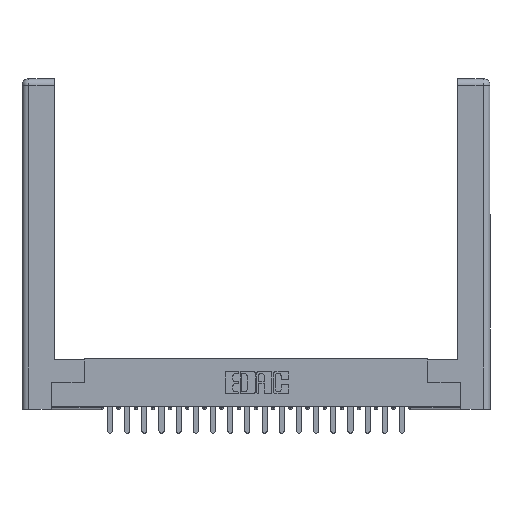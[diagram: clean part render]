
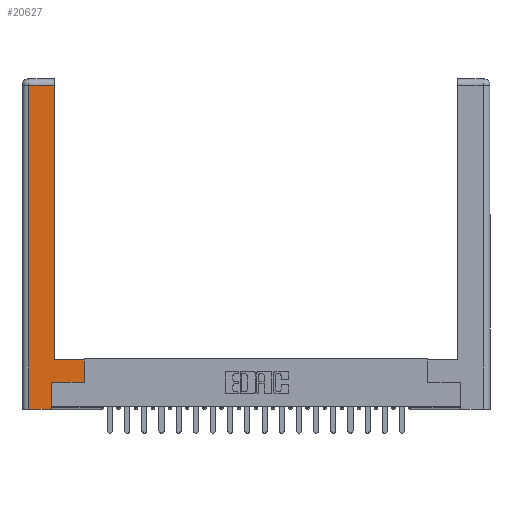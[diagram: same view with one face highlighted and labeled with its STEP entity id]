
A CAD part, top view. The second image highlights one B-rep face of the part: STEP entity #20627.
In plain terms, the highlighted planar face has unit normal (0, 0, 1).
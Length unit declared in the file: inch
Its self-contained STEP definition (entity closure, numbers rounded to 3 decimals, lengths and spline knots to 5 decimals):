
#441 = EDGE_CURVE ( 'NONE', #831, #10784, #10107, .T. ) ;
#831 = VERTEX_POINT ( 'NONE', #1088 ) ;
#875 = VERTEX_POINT ( 'NONE', #9645 ) ;
#1088 = CARTESIAN_POINT ( 'NONE',  ( 0.265, 0., 0. ) ) ;
#1110 = DIRECTION ( 'NONE',  ( 0., 1., 0. ) ) ;
#1172 = CARTESIAN_POINT ( 'NONE',  ( 0.295, 2.94, 0. ) ) ;
#2039 = ORIENTED_EDGE ( 'NONE', *, *, #11041, .T. ) ;
#2094 = EDGE_CURVE ( 'NONE', #875, #831, #14665, .T. ) ;
#2495 = LINE ( 'NONE', #18204, #14681 ) ;
#2795 = DIRECTION ( 'NONE',  ( -1., 0., 0. ) ) ;
#2903 = CARTESIAN_POINT ( 'NONE',  ( 0.295, 0.45, 0. ) ) ;
#3688 = VECTOR ( 'NONE', #4203, 39.37008 ) ;
#4203 = DIRECTION ( 'NONE',  ( 0., -1., 0. ) ) ;
#4451 = ORIENTED_EDGE ( 'NONE', *, *, #441, .T. ) ;
#4607 = EDGE_CURVE ( 'NONE', #14714, #12473, #17667, .T. ) ;
#5435 = VERTEX_POINT ( 'NONE', #10534 ) ;
#6139 = EDGE_CURVE ( 'NONE', #10784, #10225, #8619, .T. ) ;
#6574 = FACE_OUTER_BOUND ( 'NONE', #7853, .T. ) ;
#6726 = VECTOR ( 'NONE', #14790, 39.37008 ) ;
#6830 = EDGE_CURVE ( 'NONE', #12473, #5435, #9835, .T. ) ;
#7853 = EDGE_LOOP ( 'NONE', ( #19457, #12500, #12018, #20500, #4451, #14491, #15634, #2039 ) ) ;
#8029 = LINE ( 'NONE', #20234, #3688 ) ;
#8560 = VECTOR ( 'NONE', #18089, 39.37008 ) ;
#8619 = LINE ( 'NONE', #8733, #14175 ) ;
#8733 = CARTESIAN_POINT ( 'NONE',  ( 0.565, 0.245, 0. ) ) ;
#8823 = VECTOR ( 'NONE', #9847, 39.37008 ) ;
#9158 = EDGE_CURVE ( 'NONE', #5435, #875, #8029, .T. ) ;
#9365 = CARTESIAN_POINT ( 'NONE',  ( 0.295, 0.45, 0. ) ) ;
#9645 = CARTESIAN_POINT ( 'NONE',  ( 0.0615, 0., 0. ) ) ;
#9835 = LINE ( 'NONE', #20214, #10561 ) ;
#9847 = DIRECTION ( 'NONE',  ( -1., 0., 0. ) ) ;
#10107 = LINE ( 'NONE', #18434, #6726 ) ;
#10225 = VERTEX_POINT ( 'NONE', #17861 ) ;
#10534 = CARTESIAN_POINT ( 'NONE',  ( 0.0615, 2.94, 0. ) ) ;
#10561 = VECTOR ( 'NONE', #2795, 39.37008 ) ;
#10784 = VERTEX_POINT ( 'NONE', #21710 ) ;
#11041 = EDGE_CURVE ( 'NONE', #17816, #14714, #15302, .T. ) ;
#11149 = CARTESIAN_POINT ( 'NONE',  ( 0.265, 0., 0. ) ) ;
#11491 = EDGE_CURVE ( 'NONE', #10225, #17816, #2495, .T. ) ;
#11702 = DIRECTION ( 'NONE',  ( -1., 0., 0. ) ) ;
#12018 = ORIENTED_EDGE ( 'NONE', *, *, #9158, .T. ) ;
#12473 = VERTEX_POINT ( 'NONE', #1172 ) ;
#12500 = ORIENTED_EDGE ( 'NONE', *, *, #6830, .T. ) ;
#12675 = VECTOR ( 'NONE', #18348, 39.37008 ) ;
#13503 = AXIS2_PLACEMENT_3D ( 'NONE', #22280, #13642, #11702 ) ;
#13530 = PLANE ( 'NONE',  #13503 ) ;
#13642 = DIRECTION ( 'NONE',  ( 0., 0., -1. ) ) ;
#14175 = VECTOR ( 'NONE', #15678, 39.37008 ) ;
#14491 = ORIENTED_EDGE ( 'NONE', *, *, #6139, .T. ) ;
#14665 = LINE ( 'NONE', #11149, #8560 ) ;
#14681 = VECTOR ( 'NONE', #1110, 39.37008 ) ;
#14714 = VERTEX_POINT ( 'NONE', #9365 ) ;
#14790 = DIRECTION ( 'NONE',  ( 0., 1., 0. ) ) ;
#14809 = CARTESIAN_POINT ( 'NONE',  ( 0.295, 3., 0. ) ) ;
#15302 = LINE ( 'NONE', #2903, #8823 ) ;
#15634 = ORIENTED_EDGE ( 'NONE', *, *, #11491, .T. ) ;
#15678 = DIRECTION ( 'NONE',  ( 1., 0., 0. ) ) ;
#17145 = CARTESIAN_POINT ( 'NONE',  ( 0.565, 0.45, 0. ) ) ;
#17667 = LINE ( 'NONE', #14809, #12675 ) ;
#17816 = VERTEX_POINT ( 'NONE', #17145 ) ;
#17861 = CARTESIAN_POINT ( 'NONE',  ( 0.565, 0.245, 0. ) ) ;
#18089 = DIRECTION ( 'NONE',  ( 1., 0., 0. ) ) ;
#18204 = CARTESIAN_POINT ( 'NONE',  ( 0.565, 0.45, 0. ) ) ;
#18348 = DIRECTION ( 'NONE',  ( 0., 1., 0. ) ) ;
#18434 = CARTESIAN_POINT ( 'NONE',  ( 0.265, 0.245, 0. ) ) ;
#19457 = ORIENTED_EDGE ( 'NONE', *, *, #4607, .T. ) ;
#20214 = CARTESIAN_POINT ( 'NONE',  ( 0.0615, 2.94, 0. ) ) ;
#20234 = CARTESIAN_POINT ( 'NONE',  ( 0.0615, 0., 0. ) ) ;
#20500 = ORIENTED_EDGE ( 'NONE', *, *, #2094, .T. ) ;
#20627 = ADVANCED_FACE ( 'NONE', ( #6574 ), #13530, .F. ) ;
#21710 = CARTESIAN_POINT ( 'NONE',  ( 0.265, 0.245, 0. ) ) ;
#22280 = CARTESIAN_POINT ( 'NONE',  ( 0., 0., 0. ) ) ;
